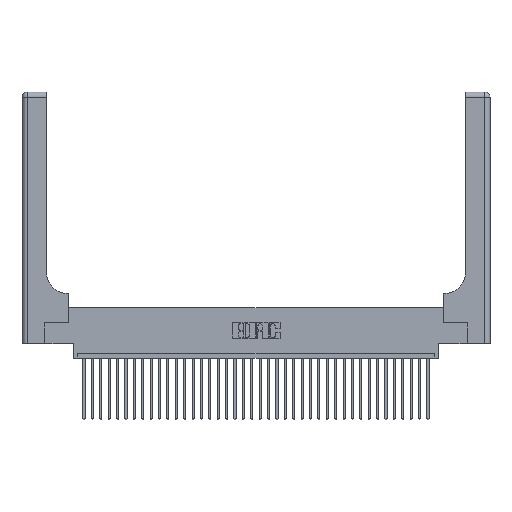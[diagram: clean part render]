
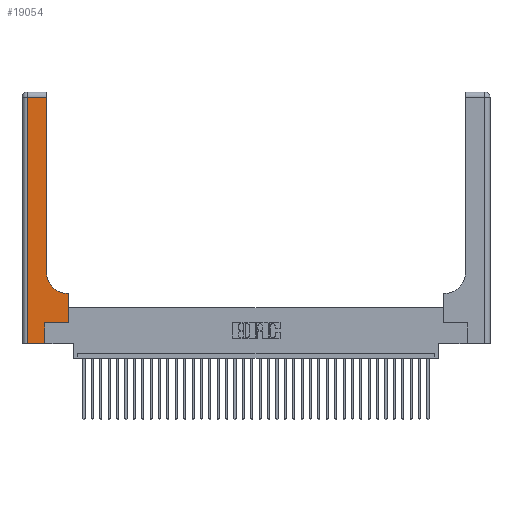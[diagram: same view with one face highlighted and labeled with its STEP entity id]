
A CAD part, top view. The second image highlights one B-rep face of the part: STEP entity #19054.
In plain terms, the highlighted planar face has unit normal (0, 0, 1).
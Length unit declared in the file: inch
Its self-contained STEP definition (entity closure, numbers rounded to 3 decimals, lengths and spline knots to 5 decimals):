
#103 = ORIENTED_EDGE ( 'NONE', *, *, #32312, .T. ) ;
#276 = PLANE ( 'NONE',  #16124 ) ;
#500 = DIRECTION ( 'NONE',  ( 1., 0., 0. ) ) ;
#828 = CARTESIAN_POINT ( 'NONE',  ( 0.06, 3., 0.37 ) ) ;
#1108 = VECTOR ( 'NONE', #5316, 39.37008 ) ;
#1647 = ORIENTED_EDGE ( 'NONE', *, *, #11144, .T. ) ;
#1792 = VECTOR ( 'NONE', #10348, 39.37008 ) ;
#1806 = EDGE_CURVE ( 'NONE', #32787, #12310, #22003, .T. ) ;
#2153 = LINE ( 'NONE', #30107, #17291 ) ;
#3520 = VERTEX_POINT ( 'NONE', #32758 ) ;
#3607 = DIRECTION ( 'NONE',  ( 0., 0., -1. ) ) ;
#4017 = DIRECTION ( 'NONE',  ( 0., 1., 0. ) ) ;
#5316 = DIRECTION ( 'NONE',  ( 0., 1., 0. ) ) ;
#5942 = EDGE_CURVE ( 'NONE', #3520, #32787, #2153, .T. ) ;
#6121 = CARTESIAN_POINT ( 'NONE',  ( 0., 3., 0.37 ) ) ;
#6687 = FACE_OUTER_BOUND ( 'NONE', #13116, .T. ) ;
#6755 = CARTESIAN_POINT ( 'NONE',  ( 0.5585, 0.6, 0.37 ) ) ;
#9102 = CARTESIAN_POINT ( 'NONE',  ( 0.269, 0., 0.37 ) ) ;
#9780 = ORIENTED_EDGE ( 'NONE', *, *, #14615, .T. ) ;
#10348 = DIRECTION ( 'NONE',  ( -1., 0., 0. ) ) ;
#11144 = EDGE_CURVE ( 'NONE', #22745, #12863, #20961, .T. ) ;
#11292 = CIRCLE ( 'NONE', #22311, 0.25 ) ;
#12310 = VERTEX_POINT ( 'NONE', #33744 ) ;
#12626 = ORIENTED_EDGE ( 'NONE', *, *, #5942, .T. ) ;
#12863 = VERTEX_POINT ( 'NONE', #17822 ) ;
#13116 = EDGE_LOOP ( 'NONE', ( #28786, #12626, #35189, #36453, #9780, #26666, #103, #1647, #32621 ) ) ;
#14615 = EDGE_CURVE ( 'NONE', #16372, #30058, #32765, .T. ) ;
#14786 = VECTOR ( 'NONE', #17766, 39.37008 ) ;
#14913 = CARTESIAN_POINT ( 'NONE',  ( 0.269, 0.25, 0.37 ) ) ;
#15233 = VECTOR ( 'NONE', #27787, 39.37008 ) ;
#15861 = CARTESIAN_POINT ( 'NONE',  ( 0.5585, 0.25, 0.37 ) ) ;
#15868 = DIRECTION ( 'NONE',  ( -1., 0., 0. ) ) ;
#16124 = AXIS2_PLACEMENT_3D ( 'NONE', #6121, #34536, #34418 ) ;
#16234 = CARTESIAN_POINT ( 'NONE',  ( 0., 0., 0.37 ) ) ;
#16372 = VERTEX_POINT ( 'NONE', #9102 ) ;
#16854 = EDGE_CURVE ( 'NONE', #30058, #33512, #20710, .T. ) ;
#16947 = EDGE_CURVE ( 'NONE', #12863, #18179, #11292, .T. ) ;
#17291 = VECTOR ( 'NONE', #15868, 39.37008 ) ;
#17766 = DIRECTION ( 'NONE',  ( 0., -1., 0. ) ) ;
#17822 = CARTESIAN_POINT ( 'NONE',  ( 0.5415, 0.6, 0.37 ) ) ;
#18179 = VERTEX_POINT ( 'NONE', #22161 ) ;
#18864 = CARTESIAN_POINT ( 'NONE',  ( 0.2915, 0.6, 0.37 ) ) ;
#19054 = ADVANCED_FACE ( 'NONE', ( #6687 ), #276, .F. ) ;
#19263 = DIRECTION ( 'NONE',  ( 1., 0., 0. ) ) ;
#20710 = LINE ( 'NONE', #14913, #30558 ) ;
#20961 = LINE ( 'NONE', #18864, #1792 ) ;
#22003 = LINE ( 'NONE', #828, #14786 ) ;
#22161 = CARTESIAN_POINT ( 'NONE',  ( 0.2915, 0.85, 0.37 ) ) ;
#22311 = AXIS2_PLACEMENT_3D ( 'NONE', #28760, #3607, #34506 ) ;
#22745 = VERTEX_POINT ( 'NONE', #6755 ) ;
#23298 = LINE ( 'NONE', #24810, #15233 ) ;
#24072 = CARTESIAN_POINT ( 'NONE',  ( 0.2915, 3., 0.37 ) ) ;
#24810 = CARTESIAN_POINT ( 'NONE',  ( 0.5585, 0.25, 0.37 ) ) ;
#26666 = ORIENTED_EDGE ( 'NONE', *, *, #16854, .T. ) ;
#27169 = CARTESIAN_POINT ( 'NONE',  ( 0.269, 0., 0.37 ) ) ;
#27787 = DIRECTION ( 'NONE',  ( 0., 1., 0. ) ) ;
#28531 = LINE ( 'NONE', #16234, #29936 ) ;
#28760 = CARTESIAN_POINT ( 'NONE',  ( 0.5415, 0.85, 0.37 ) ) ;
#28786 = ORIENTED_EDGE ( 'NONE', *, *, #31076, .T. ) ;
#29936 = VECTOR ( 'NONE', #19263, 39.37008 ) ;
#30058 = VERTEX_POINT ( 'NONE', #33381 ) ;
#30107 = CARTESIAN_POINT ( 'NONE',  ( 0., 2.94, 0.37 ) ) ;
#30558 = VECTOR ( 'NONE', #500, 39.37008 ) ;
#30593 = EDGE_CURVE ( 'NONE', #12310, #16372, #28531, .T. ) ;
#31076 = EDGE_CURVE ( 'NONE', #18179, #3520, #36557, .T. ) ;
#32312 = EDGE_CURVE ( 'NONE', #33512, #22745, #23298, .T. ) ;
#32621 = ORIENTED_EDGE ( 'NONE', *, *, #16947, .T. ) ;
#32758 = CARTESIAN_POINT ( 'NONE',  ( 0.2915, 2.94, 0.37 ) ) ;
#32765 = LINE ( 'NONE', #27169, #1108 ) ;
#32787 = VERTEX_POINT ( 'NONE', #35494 ) ;
#33017 = VECTOR ( 'NONE', #4017, 39.37008 ) ;
#33381 = CARTESIAN_POINT ( 'NONE',  ( 0.269, 0.25, 0.37 ) ) ;
#33512 = VERTEX_POINT ( 'NONE', #15861 ) ;
#33744 = CARTESIAN_POINT ( 'NONE',  ( 0.06, 0., 0.37 ) ) ;
#34418 = DIRECTION ( 'NONE',  ( -1., 0., 0. ) ) ;
#34506 = DIRECTION ( 'NONE',  ( 1., 0., 0. ) ) ;
#34536 = DIRECTION ( 'NONE',  ( 0., 0., -1. ) ) ;
#35189 = ORIENTED_EDGE ( 'NONE', *, *, #1806, .T. ) ;
#35494 = CARTESIAN_POINT ( 'NONE',  ( 0.06, 2.94, 0.37 ) ) ;
#36453 = ORIENTED_EDGE ( 'NONE', *, *, #30593, .T. ) ;
#36557 = LINE ( 'NONE', #24072, #33017 ) ;
